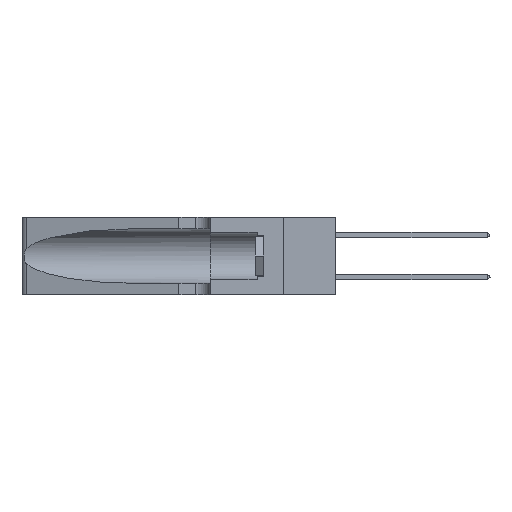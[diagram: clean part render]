
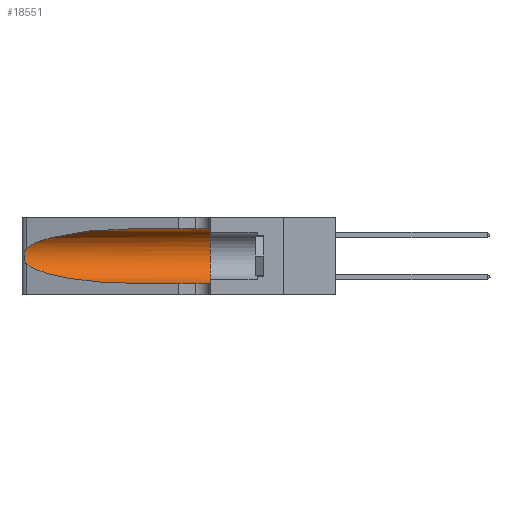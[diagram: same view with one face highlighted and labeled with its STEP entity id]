
A CAD part, left-side view. The second image highlights one B-rep face of the part: STEP entity #18551.
In plain terms, the highlighted cylindrical face has radius 3.308 mm (diameter 6.617 mm), a partial arc.
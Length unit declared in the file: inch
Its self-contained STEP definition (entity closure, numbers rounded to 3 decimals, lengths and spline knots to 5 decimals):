
#1323 = EDGE_LOOP ( 'NONE', ( #6415, #2783, #20018, #23373, #14166, #3824 ) ) ;
#1502 = CARTESIAN_POINT ( 'NONE',  ( 0.25487, 1.22718, 0.22369 ) ) ;
#1949 = VERTEX_POINT ( 'NONE', #11942 ) ;
#2147 = EDGE_CURVE ( 'NONE', #24820, #13603, #6904, .T. ) ;
#2183 = VECTOR ( 'NONE', #24150, 39.37008 ) ;
#2757 = CARTESIAN_POINT ( 'NONE',  ( 0.26075, 1.23896, 0.178 ) ) ;
#2783 = ORIENTED_EDGE ( 'NONE', *, *, #7020, .T. ) ;
#3463 = CARTESIAN_POINT ( 'NONE',  ( 0.25487, 1.22718, 0.14631 ) ) ;
#3466 = AXIS2_PLACEMENT_3D ( 'NONE', #22293, #25005, #10301 ) ;
#3824 = ORIENTED_EDGE ( 'NONE', *, *, #20504, .F. ) ;
#4094 = LINE ( 'NONE', #18334, #2183 ) ;
#4273 = EDGE_CURVE ( 'NONE', #26165, #8279, #4584, .T. ) ;
#4584 = CIRCLE ( 'NONE', #3466, 0.13025 ) ;
#4910 = CARTESIAN_POINT ( 'NONE',  ( 0.1305, 0.35, 0.31525 ) ) ;
#5047 = CARTESIAN_POINT ( 'NONE',  ( 0.1305, 1.61858, 0.31525 ) ) ;
#5499 = EDGE_CURVE ( 'NONE', #30118, #8279, #4094, .T. ) ;
#6415 = ORIENTED_EDGE ( 'NONE', *, *, #2147, .T. ) ;
#6673 = CARTESIAN_POINT ( 'NONE',  ( 0.1305, 0.72297, 0.05475 ) ) ;
#6904 =( BOUNDED_CURVE ( )  B_SPLINE_CURVE ( 3, ( #30745, #8186, #23859, #30414 ),
 .UNSPECIFIED., .F., .F. ) 
 B_SPLINE_CURVE_WITH_KNOTS ( ( 4, 4 ),
 ( 1.5708, 2.84003 ),
 .UNSPECIFIED. ) 
 CURVE ( )  GEOMETRIC_REPRESENTATION_ITEM ( )  RATIONAL_B_SPLINE_CURVE ( ( 1., 0.87, 0.87, 1. ) ) 
 REPRESENTATION_ITEM ( '' )  );
#7020 = EDGE_CURVE ( 'NONE', #13603, #1949, #25071, .T. ) ;
#8186 = CARTESIAN_POINT ( 'NONE',  ( 0.18966, 0.96281, 0.31525 ) ) ;
#8279 = VERTEX_POINT ( 'NONE', #14475 ) ;
#9742 = AXIS2_PLACEMENT_3D ( 'NONE', #22535, #27405, #12593 ) ;
#10048 = FACE_OUTER_BOUND ( 'NONE', #1323, .T. ) ;
#10301 = DIRECTION ( 'NONE',  ( 0., 0., 1. ) ) ;
#11041 = CARTESIAN_POINT ( 'NONE',  ( 0.2373, 1.15595, 0.08982 ) ) ;
#11043 = CARTESIAN_POINT ( 'NONE',  ( 0.1305, 0.72297, 0.31525 ) ) ;
#11287 = VECTOR ( 'NONE', #12527, 39.37008 ) ;
#11942 = CARTESIAN_POINT ( 'NONE',  ( 0.25487, 1.22718, 0.14631 ) ) ;
#12527 = DIRECTION ( 'NONE',  ( 0., -1., 0. ) ) ;
#12593 = DIRECTION ( 'NONE',  ( 0., 0., -1. ) ) ;
#13603 = VERTEX_POINT ( 'NONE', #31372 ) ;
#14166 = ORIENTED_EDGE ( 'NONE', *, *, #4273, .F. ) ;
#14475 = CARTESIAN_POINT ( 'NONE',  ( 0.1305, 0.35, 0.05475 ) ) ;
#15112 = CARTESIAN_POINT ( 'NONE',  ( 0.25639, 1.23184, 0.21858 ) ) ;
#15115 = CARTESIAN_POINT ( 'NONE',  ( 0.26017, 1.23833, 0.17102 ) ) ;
#15808 = CYLINDRICAL_SURFACE ( 'NONE', #9742, 0.13025 ) ;
#16278 = CARTESIAN_POINT ( 'NONE',  ( 0.1305, 0.72297, 0.05475 ) ) ;
#16286 = CARTESIAN_POINT ( 'NONE',  ( 0.26018, 1.23835, 0.19895 ) ) ;
#18121 = CARTESIAN_POINT ( 'NONE',  ( 0.25854, 1.2359, 0.20912 ) ) ;
#18334 = CARTESIAN_POINT ( 'NONE',  ( 0.1305, 1.61858, 0.05475 ) ) ;
#18551 = ADVANCED_FACE ( 'NONE', ( #10048 ), #15808, .F. ) ;
#19729 = EDGE_CURVE ( 'NONE', #1949, #30118, #27418, .T. ) ;
#20018 = ORIENTED_EDGE ( 'NONE', *, *, #19729, .T. ) ;
#20504 = EDGE_CURVE ( 'NONE', #24820, #26165, #23674, .T. ) ;
#20802 = CARTESIAN_POINT ( 'NONE',  ( 0.25639, 1.23186, 0.15144 ) ) ;
#22293 = CARTESIAN_POINT ( 'NONE',  ( 0.1305, 0.35, 0.185 ) ) ;
#22535 = CARTESIAN_POINT ( 'NONE',  ( 0.1305, 1.61858, 0.185 ) ) ;
#23270 = CARTESIAN_POINT ( 'NONE',  ( 0.25789, 1.23486, 0.15765 ) ) ;
#23317 = CARTESIAN_POINT ( 'NONE',  ( 0.25487, 1.22718, 0.14631 ) ) ;
#23373 = ORIENTED_EDGE ( 'NONE', *, *, #5499, .T. ) ;
#23674 = LINE ( 'NONE', #5047, #11287 ) ;
#23859 = CARTESIAN_POINT ( 'NONE',  ( 0.2373, 1.15595, 0.28018 ) ) ;
#24150 = DIRECTION ( 'NONE',  ( 0., -1., 0. ) ) ;
#24820 = VERTEX_POINT ( 'NONE', #11043 ) ;
#25005 = DIRECTION ( 'NONE',  ( 0., 1., 0. ) ) ;
#25071 = B_SPLINE_CURVE_WITH_KNOTS ( 'NONE', 3,
 ( #1502, #27834, #15112, #30243, #18121, #16286, #25892, #2757, #15115, #25100, #23270, #20802, #26028, #3463 ),
 .UNSPECIFIED., .F., .F.,
 ( 4, 2, 2, 2, 2, 2, 4 ),
 ( 0., 0.00027, 0.00053, 0.00107, 0.0016, 0.00187, 0.00214 ),
 .UNSPECIFIED. ) ;
#25100 = CARTESIAN_POINT ( 'NONE',  ( 0.25856, 1.23593, 0.16098 ) ) ;
#25892 = CARTESIAN_POINT ( 'NONE',  ( 0.26075, 1.23896, 0.19203 ) ) ;
#26028 = CARTESIAN_POINT ( 'NONE',  ( 0.25555, 1.22993, 0.14849 ) ) ;
#26165 = VERTEX_POINT ( 'NONE', #4910 ) ;
#27405 = DIRECTION ( 'NONE',  ( 0., -1., 0. ) ) ;
#27418 =( BOUNDED_CURVE ( )  B_SPLINE_CURVE ( 3, ( #23317, #11041, #30925, #6673 ),
 .UNSPECIFIED., .F., .T. ) 
 B_SPLINE_CURVE_WITH_KNOTS ( ( 4, 4 ),
 ( 3.44316, 4.71239 ),
 .UNSPECIFIED. ) 
 CURVE ( )  GEOMETRIC_REPRESENTATION_ITEM ( )  RATIONAL_B_SPLINE_CURVE ( ( 1., 0.87, 0.87, 1. ) ) 
 REPRESENTATION_ITEM ( '' )  );
#27834 = CARTESIAN_POINT ( 'NONE',  ( 0.25555, 1.22994, 0.2215 ) ) ;
#30118 = VERTEX_POINT ( 'NONE', #16278 ) ;
#30243 = CARTESIAN_POINT ( 'NONE',  ( 0.25787, 1.23484, 0.2124 ) ) ;
#30414 = CARTESIAN_POINT ( 'NONE',  ( 0.25487, 1.22718, 0.22369 ) ) ;
#30745 = CARTESIAN_POINT ( 'NONE',  ( 0.1305, 0.72297, 0.31525 ) ) ;
#30925 = CARTESIAN_POINT ( 'NONE',  ( 0.18966, 0.96281, 0.05475 ) ) ;
#31372 = CARTESIAN_POINT ( 'NONE',  ( 0.25487, 1.22718, 0.22369 ) ) ;
